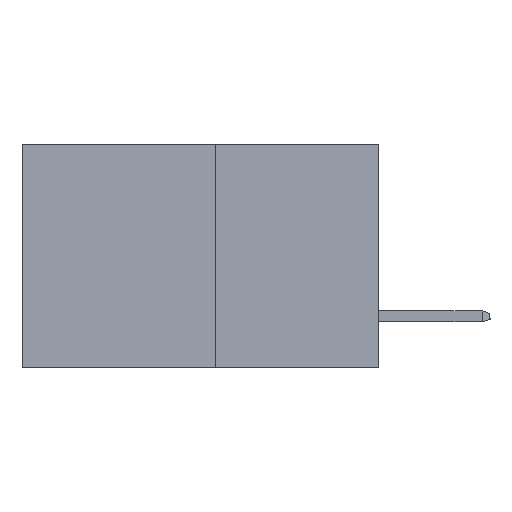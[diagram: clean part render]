
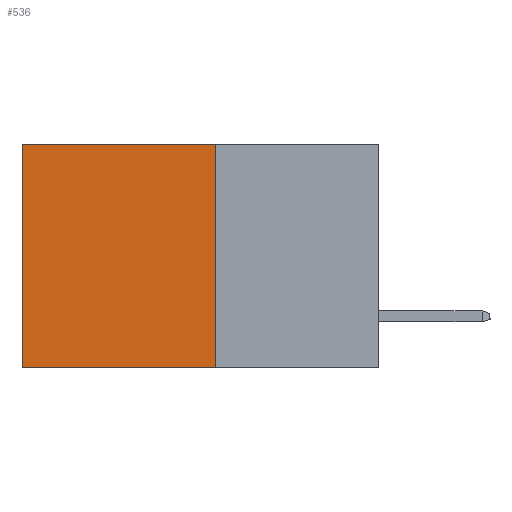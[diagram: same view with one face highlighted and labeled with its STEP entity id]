
A CAD part, left-side view. The second image highlights one B-rep face of the part: STEP entity #536.
In plain terms, the highlighted planar face has unit normal (-1, 0, 0).
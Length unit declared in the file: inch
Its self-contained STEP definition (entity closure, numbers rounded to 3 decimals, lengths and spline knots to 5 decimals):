
#129 = DIRECTION ( 'NONE',  ( 0., 0., -1. ) ) ;
#173 = VERTEX_POINT ( 'NONE', #10632 ) ;
#536 = ADVANCED_FACE ( 'NONE', ( #6653 ), #2122, .F. ) ;
#772 = DIRECTION ( 'NONE',  ( 1., 0., 0. ) ) ;
#1441 = CARTESIAN_POINT ( 'NONE',  ( 0.277, 0.27, -0.37 ) ) ;
#1610 = VECTOR ( 'NONE', #9010, 39.37008 ) ;
#1666 = ORIENTED_EDGE ( 'NONE', *, *, #3616, .F. ) ;
#2122 = PLANE ( 'NONE',  #4221 ) ;
#2179 = VERTEX_POINT ( 'NONE', #5860 ) ;
#2212 = ORIENTED_EDGE ( 'NONE', *, *, #4905, .T. ) ;
#2383 = VECTOR ( 'NONE', #7317, 39.37008 ) ;
#2409 = EDGE_CURVE ( 'NONE', #173, #2179, #5259, .T. ) ;
#2674 = CARTESIAN_POINT ( 'NONE',  ( 0.277, 0.27, -0.37 ) ) ;
#3616 = EDGE_CURVE ( 'NONE', #10181, #173, #9294, .T. ) ;
#3687 = EDGE_CURVE ( 'NONE', #8607, #2179, #11315, .T. ) ;
#4221 = AXIS2_PLACEMENT_3D ( 'NONE', #1441, #772, #129 ) ;
#4905 = EDGE_CURVE ( 'NONE', #10181, #8607, #10060, .T. ) ;
#5259 = LINE ( 'NONE', #2674, #2383 ) ;
#5860 = CARTESIAN_POINT ( 'NONE',  ( 0.277, 0.59, -0.37 ) ) ;
#6509 = CARTESIAN_POINT ( 'NONE',  ( 0.277, 0.27, -0.37 ) ) ;
#6535 = VECTOR ( 'NONE', #11666, 39.37008 ) ;
#6653 = FACE_OUTER_BOUND ( 'NONE', #7919, .T. ) ;
#7317 = DIRECTION ( 'NONE',  ( 0., 1., 0. ) ) ;
#7338 = CARTESIAN_POINT ( 'NONE',  ( 0.277, 0.59, 0. ) ) ;
#7919 = EDGE_LOOP ( 'NONE', ( #11848, #8528, #1666, #2212 ) ) ;
#8023 = DIRECTION ( 'NONE',  ( 0., 0., -1. ) ) ;
#8528 = ORIENTED_EDGE ( 'NONE', *, *, #2409, .F. ) ;
#8607 = VERTEX_POINT ( 'NONE', #7338 ) ;
#8934 = CARTESIAN_POINT ( 'NONE',  ( 0.277, 0.27, 0. ) ) ;
#9010 = DIRECTION ( 'NONE',  ( 0., 1., 0. ) ) ;
#9294 = LINE ( 'NONE', #6509, #6535 ) ;
#9983 = CARTESIAN_POINT ( 'NONE',  ( 0.277, 0.27, 0. ) ) ;
#10060 = LINE ( 'NONE', #8934, #1610 ) ;
#10181 = VERTEX_POINT ( 'NONE', #9983 ) ;
#10632 = CARTESIAN_POINT ( 'NONE',  ( 0.277, 0.27, -0.37 ) ) ;
#11003 = VECTOR ( 'NONE', #8023, 39.37008 ) ;
#11315 = LINE ( 'NONE', #11954, #11003 ) ;
#11666 = DIRECTION ( 'NONE',  ( 0., 0., -1. ) ) ;
#11848 = ORIENTED_EDGE ( 'NONE', *, *, #3687, .T. ) ;
#11954 = CARTESIAN_POINT ( 'NONE',  ( 0.277, 0.59, -0.37 ) ) ;
